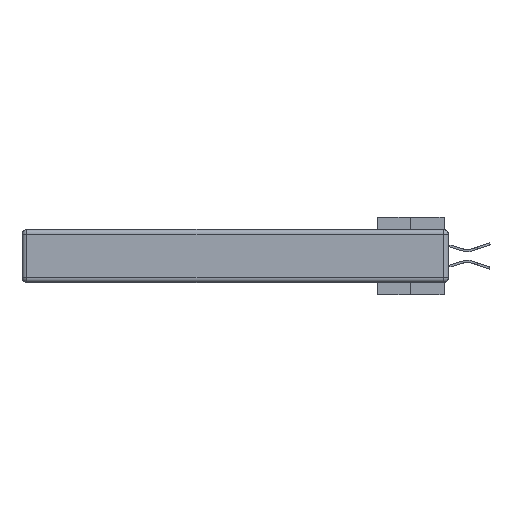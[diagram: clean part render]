
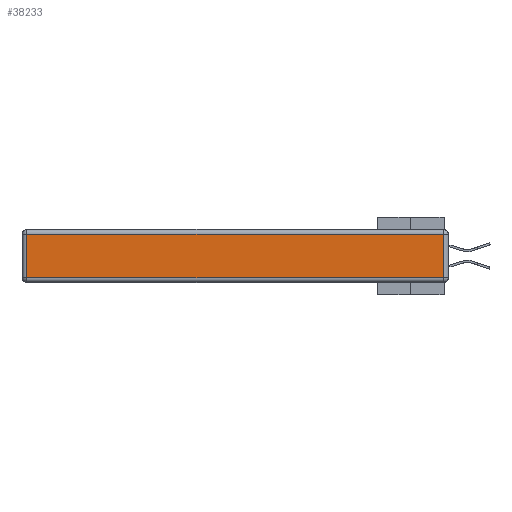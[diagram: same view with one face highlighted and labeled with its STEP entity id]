
A CAD part, left-side view. The second image highlights one B-rep face of the part: STEP entity #38233.
In plain terms, the highlighted planar face has unit normal (-1, 0, 0).
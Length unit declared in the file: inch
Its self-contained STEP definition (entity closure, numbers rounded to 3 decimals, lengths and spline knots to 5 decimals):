
#151 = DIRECTION ( 'NONE',  ( 0., 0., -1. ) ) ;
#335 = VERTEX_POINT ( 'NONE', #12843 ) ;
#2630 = CARTESIAN_POINT ( 'NONE',  ( 0., 2.72, -0.313 ) ) ;
#5626 = CARTESIAN_POINT ( 'NONE',  ( 0., 2.72, -0.03 ) ) ;
#6292 = ORIENTED_EDGE ( 'NONE', *, *, #18798, .T. ) ;
#6502 = DIRECTION ( 'NONE',  ( 0., 0., 1. ) ) ;
#6706 = VECTOR ( 'NONE', #22725, 39.37008 ) ;
#7115 = EDGE_CURVE ( 'NONE', #335, #37480, #9361, .T. ) ;
#7342 = DIRECTION ( 'NONE',  ( 0., -1., 0. ) ) ;
#9361 = LINE ( 'NONE', #32322, #6706 ) ;
#9948 = FACE_OUTER_BOUND ( 'NONE', #35719, .T. ) ;
#11401 = LINE ( 'NONE', #23656, #15050 ) ;
#12843 = CARTESIAN_POINT ( 'NONE',  ( 0., 0.03, -0.03 ) ) ;
#15050 = VECTOR ( 'NONE', #37271, 39.37008 ) ;
#18798 = EDGE_CURVE ( 'NONE', #37480, #35304, #31485, .T. ) ;
#18854 = EDGE_CURVE ( 'NONE', #29522, #335, #11401, .T. ) ;
#19571 = EDGE_CURVE ( 'NONE', #35304, #29522, #21419, .T. ) ;
#21419 = LINE ( 'NONE', #37730, #43229 ) ;
#22725 = DIRECTION ( 'NONE',  ( 0., 1., 0. ) ) ;
#23656 = CARTESIAN_POINT ( 'NONE',  ( 0., 0.03, -0.343 ) ) ;
#25115 = VECTOR ( 'NONE', #151, 39.37008 ) ;
#25147 = CARTESIAN_POINT ( 'NONE',  ( 0., 2.72, -0.343 ) ) ;
#26767 = CARTESIAN_POINT ( 'NONE',  ( 0., 0., -0.343 ) ) ;
#29522 = VERTEX_POINT ( 'NONE', #41978 ) ;
#31042 = ORIENTED_EDGE ( 'NONE', *, *, #19571, .T. ) ;
#31485 = LINE ( 'NONE', #25147, #25115 ) ;
#32322 = CARTESIAN_POINT ( 'NONE',  ( 0., 2.75, -0.03 ) ) ;
#33344 = PLANE ( 'NONE',  #39564 ) ;
#34725 = ORIENTED_EDGE ( 'NONE', *, *, #7115, .T. ) ;
#35304 = VERTEX_POINT ( 'NONE', #2630 ) ;
#35719 = EDGE_LOOP ( 'NONE', ( #31042, #40583, #34725, #6292 ) ) ;
#37271 = DIRECTION ( 'NONE',  ( 0., 0., 1. ) ) ;
#37480 = VERTEX_POINT ( 'NONE', #5626 ) ;
#37730 = CARTESIAN_POINT ( 'NONE',  ( 0., 0., -0.313 ) ) ;
#38233 = ADVANCED_FACE ( 'NONE', ( #9948 ), #33344, .T. ) ;
#39564 = AXIS2_PLACEMENT_3D ( 'NONE', #26767, #43349, #6502 ) ;
#40583 = ORIENTED_EDGE ( 'NONE', *, *, #18854, .T. ) ;
#41978 = CARTESIAN_POINT ( 'NONE',  ( 0., 0.03, -0.313 ) ) ;
#43229 = VECTOR ( 'NONE', #7342, 39.37008 ) ;
#43349 = DIRECTION ( 'NONE',  ( -1., 0., 0. ) ) ;
